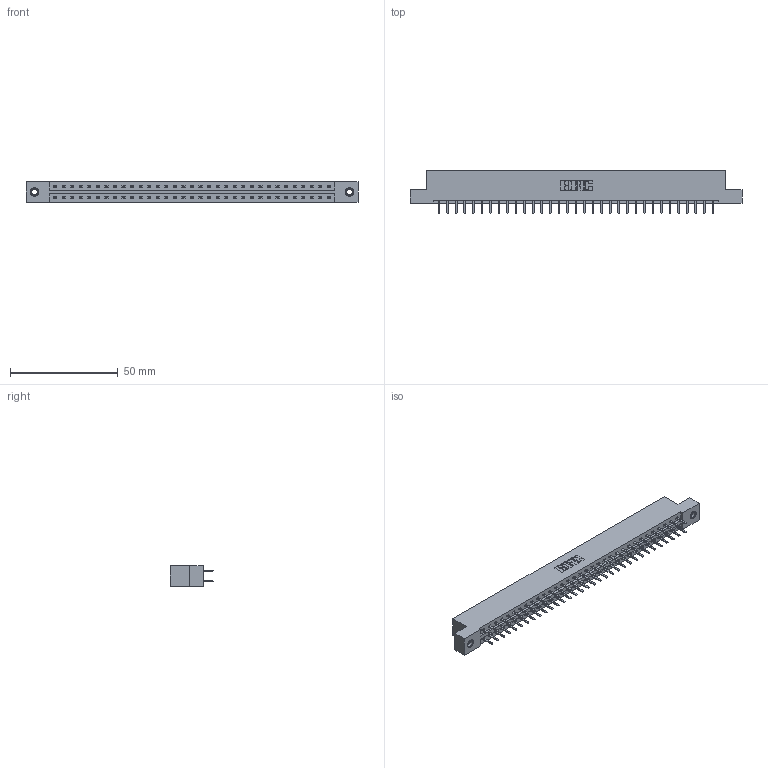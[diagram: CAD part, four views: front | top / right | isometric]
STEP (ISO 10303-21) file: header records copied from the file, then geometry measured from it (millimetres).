
FILE_DESCRIPTION (( 'STEP AP203' ), '1' );
FILE_NAME ('337-066-520-207.STEP', '2019-10-09T22:53:04', ( '' ), ( '' ), 'SwSTEP 2.0', 'SolidWorks 2016', '' );
FILE_SCHEMA (( 'CONFIG_CONTROL_DESIGN' ));
Length unit declared in the file: inch
Products named in the file (4): 337-066-520-207; 337 Part_Flush Mounting Lugs - 0.156 Dia-TI; 345-250-001_345-250-005-103; 345-292-001_345-293-120
Assembly tree (69 placements, depth 2):
  337-066-520-207
    337 Part_Flush Mounting Lugs - 0.156 Dia-TI
    345-292-001_345-293-120  x66
    345-250-001_345-250-005-103  x2
Bounding box: 153.77 x 20.02 x 9.4 mm (x, y, z)
Volume: 16043.3 mm3; surface area: 18002.8 mm2
Topology: 69 solids, 69 shells, 4002 faces, 11601 edges, 7550 vertices
Faces by surface type: plane 2742, cylinder 1244, cone 12, torus 4
Entity records: 28050 total; most frequent: CARTESIAN_POINT 4725, ORIENTED_EDGE 4642, DIRECTION 4055, EDGE_CURVE 2321, VECTOR 2169, LINE 2169, VERTEX_POINT 1540, AXIS2_PLACEMENT_3D 943
